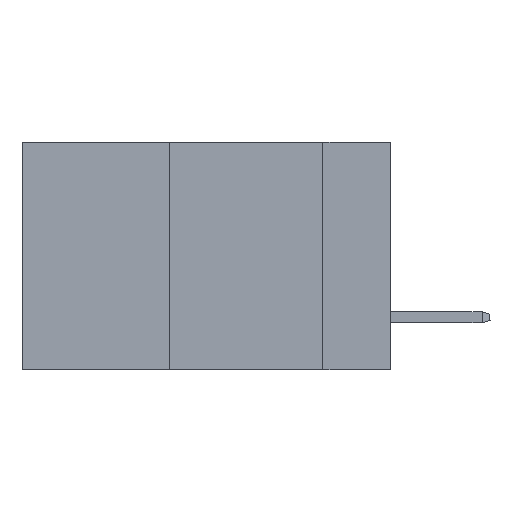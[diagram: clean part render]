
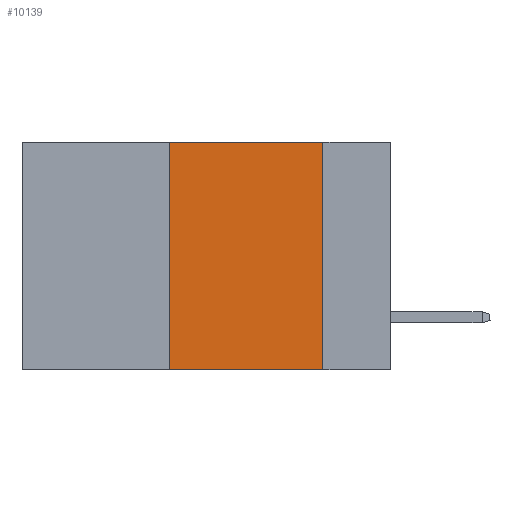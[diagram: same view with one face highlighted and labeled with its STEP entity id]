
A CAD part, left-side view. The second image highlights one B-rep face of the part: STEP entity #10139.
In plain terms, the highlighted planar face has unit normal (-1, 0, 0).
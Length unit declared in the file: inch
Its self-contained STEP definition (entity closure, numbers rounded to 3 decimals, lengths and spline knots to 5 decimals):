
#43 = ORIENTED_EDGE ( 'NONE', *, *, #6879, .F. ) ;
#722 = AXIS2_PLACEMENT_3D ( 'NONE', #5051, #7137, #1606 ) ;
#1380 = ORIENTED_EDGE ( 'NONE', *, *, #2587, .F. ) ;
#1391 = CARTESIAN_POINT ( 'NONE',  ( 0., 0.36, 0. ) ) ;
#1606 = DIRECTION ( 'NONE',  ( 0., 0., -1. ) ) ;
#2034 = EDGE_CURVE ( 'NONE', #9200, #10929, #10172, .T. ) ;
#2587 = EDGE_CURVE ( 'NONE', #10929, #7848, #10154, .T. ) ;
#2767 = CARTESIAN_POINT ( 'NONE',  ( 0., 0.11, -0.37 ) ) ;
#3282 = LINE ( 'NONE', #6378, #10092 ) ;
#3300 = DIRECTION ( 'NONE',  ( 0., 0., -1. ) ) ;
#3506 = EDGE_LOOP ( 'NONE', ( #1380, #10447, #43, #6640 ) ) ;
#4571 = CARTESIAN_POINT ( 'NONE',  ( 0., 0.6, 0. ) ) ;
#5051 = CARTESIAN_POINT ( 'NONE',  ( 0., 0.6, 0. ) ) ;
#5216 = PLANE ( 'NONE',  #722 ) ;
#5457 = LINE ( 'NONE', #10842, #5907 ) ;
#5488 = VECTOR ( 'NONE', #3300, 39.37008 ) ;
#5511 = VECTOR ( 'NONE', #10047, 39.37008 ) ;
#5907 = VECTOR ( 'NONE', #11776, 39.37008 ) ;
#6175 = EDGE_CURVE ( 'NONE', #7107, #7848, #5457, .T. ) ;
#6378 = CARTESIAN_POINT ( 'NONE',  ( 0., 0.36, 0. ) ) ;
#6640 = ORIENTED_EDGE ( 'NONE', *, *, #6175, .T. ) ;
#6879 = EDGE_CURVE ( 'NONE', #7107, #9200, #3282, .T. ) ;
#7107 = VERTEX_POINT ( 'NONE', #8930 ) ;
#7118 = FACE_OUTER_BOUND ( 'NONE', #3506, .T. ) ;
#7137 = DIRECTION ( 'NONE',  ( 1., 0., 0. ) ) ;
#7152 = CARTESIAN_POINT ( 'NONE',  ( 0., 0.11, 0. ) ) ;
#7848 = VERTEX_POINT ( 'NONE', #2767 ) ;
#8930 = CARTESIAN_POINT ( 'NONE',  ( 0., 0.36, -0.37 ) ) ;
#9200 = VERTEX_POINT ( 'NONE', #1391 ) ;
#9239 = CARTESIAN_POINT ( 'NONE',  ( 0., 0.11, 0. ) ) ;
#10047 = DIRECTION ( 'NONE',  ( 0., -1., 0. ) ) ;
#10092 = VECTOR ( 'NONE', #11941, 39.37008 ) ;
#10139 = ADVANCED_FACE ( 'NONE', ( #7118 ), #5216, .F. ) ;
#10154 = LINE ( 'NONE', #7152, #5488 ) ;
#10172 = LINE ( 'NONE', #4571, #5511 ) ;
#10447 = ORIENTED_EDGE ( 'NONE', *, *, #2034, .F. ) ;
#10842 = CARTESIAN_POINT ( 'NONE',  ( 0., 0.6, -0.37 ) ) ;
#10929 = VERTEX_POINT ( 'NONE', #9239 ) ;
#11776 = DIRECTION ( 'NONE',  ( 0., -1., 0. ) ) ;
#11941 = DIRECTION ( 'NONE',  ( 0., 0., 1. ) ) ;
